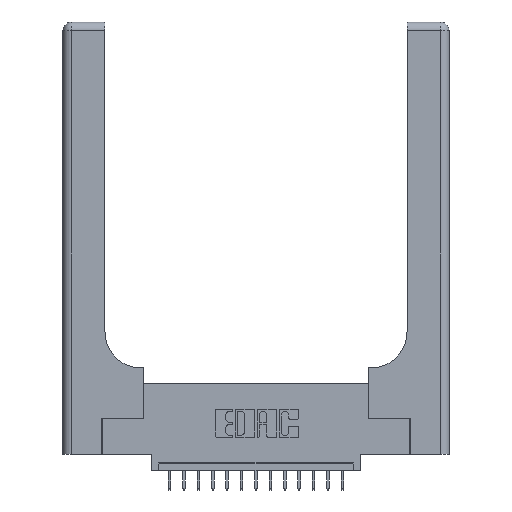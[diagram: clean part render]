
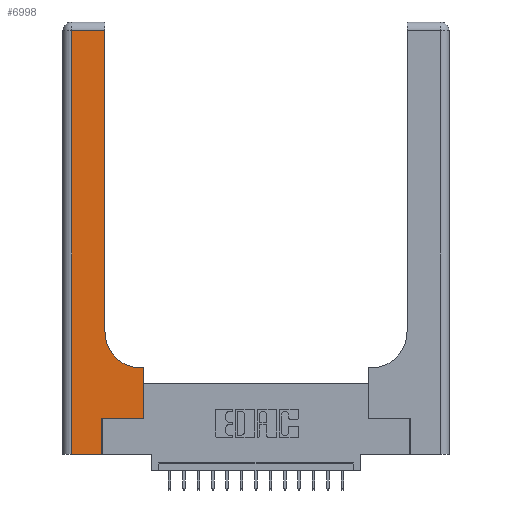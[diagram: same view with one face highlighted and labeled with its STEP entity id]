
A CAD part, top view. The second image highlights one B-rep face of the part: STEP entity #6998.
In plain terms, the highlighted planar face has unit normal (0, 0, 1).
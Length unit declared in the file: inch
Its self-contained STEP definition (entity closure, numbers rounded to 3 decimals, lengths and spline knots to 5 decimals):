
#561 = CARTESIAN_POINT ( 'NONE',  ( 0.269, 0.25, 0.37 ) ) ;
#608 = LINE ( 'NONE', #16810, #2091 ) ;
#616 = CARTESIAN_POINT ( 'NONE',  ( 0.2915, 2.94, 0.37 ) ) ;
#638 = LINE ( 'NONE', #5165, #14674 ) ;
#771 = ORIENTED_EDGE ( 'NONE', *, *, #9274, .T. ) ;
#991 = ORIENTED_EDGE ( 'NONE', *, *, #13420, .T. ) ;
#998 = ORIENTED_EDGE ( 'NONE', *, *, #8597, .T. ) ;
#1285 = DIRECTION ( 'NONE',  ( 1., 0., 0. ) ) ;
#1590 = CARTESIAN_POINT ( 'NONE',  ( 0., 2.94, 0.37 ) ) ;
#1772 = EDGE_CURVE ( 'NONE', #9181, #18291, #14982, .T. ) ;
#2091 = VECTOR ( 'NONE', #5419, 39.37008 ) ;
#2527 = FACE_OUTER_BOUND ( 'NONE', #10861, .T. ) ;
#2528 = CARTESIAN_POINT ( 'NONE',  ( 0.5585, 0.25, 0.37 ) ) ;
#2594 = EDGE_CURVE ( 'NONE', #7961, #16910, #15760, .T. ) ;
#2652 = CARTESIAN_POINT ( 'NONE',  ( 0., 0., 0.37 ) ) ;
#2973 = DIRECTION ( 'NONE',  ( 1., 0., 0. ) ) ;
#2987 = ORIENTED_EDGE ( 'NONE', *, *, #18652, .T. ) ;
#3195 = DIRECTION ( 'NONE',  ( 0., 1., 0. ) ) ;
#3884 = CIRCLE ( 'NONE', #10097, 0.25 ) ;
#4090 = LINE ( 'NONE', #9847, #17593 ) ;
#4193 = VERTEX_POINT ( 'NONE', #12497 ) ;
#4976 = CARTESIAN_POINT ( 'NONE',  ( 0.269, 0., 0.37 ) ) ;
#5077 = VECTOR ( 'NONE', #7003, 39.37008 ) ;
#5145 = CARTESIAN_POINT ( 'NONE',  ( 0.5585, 0.6, 0.37 ) ) ;
#5165 = CARTESIAN_POINT ( 'NONE',  ( 0.2915, 0.6, 0.37 ) ) ;
#5419 = DIRECTION ( 'NONE',  ( 0., 1., 0. ) ) ;
#5453 = VERTEX_POINT ( 'NONE', #616 ) ;
#6640 = AXIS2_PLACEMENT_3D ( 'NONE', #7092, #8457, #6906 ) ;
#6906 = DIRECTION ( 'NONE',  ( -1., 0., 0. ) ) ;
#6998 = ADVANCED_FACE ( 'NONE', ( #2527 ), #13167, .F. ) ;
#7003 = DIRECTION ( 'NONE',  ( 0., 1., 0. ) ) ;
#7092 = CARTESIAN_POINT ( 'NONE',  ( 0., 3., 0.37 ) ) ;
#7511 = DIRECTION ( 'NONE',  ( -1., 0., 0. ) ) ;
#7774 = VECTOR ( 'NONE', #7511, 39.37008 ) ;
#7961 = VERTEX_POINT ( 'NONE', #15566 ) ;
#8004 = DIRECTION ( 'NONE',  ( -1., 0., 0. ) ) ;
#8240 = CARTESIAN_POINT ( 'NONE',  ( 0.5415, 0.6, 0.37 ) ) ;
#8259 = ORIENTED_EDGE ( 'NONE', *, *, #2594, .T. ) ;
#8457 = DIRECTION ( 'NONE',  ( 0., 0., -1. ) ) ;
#8597 = EDGE_CURVE ( 'NONE', #17980, #13840, #3884, .T. ) ;
#8748 = VERTEX_POINT ( 'NONE', #13701 ) ;
#9069 = LINE ( 'NONE', #1590, #7774 ) ;
#9181 = VERTEX_POINT ( 'NONE', #4976 ) ;
#9274 = EDGE_CURVE ( 'NONE', #16910, #17980, #638, .T. ) ;
#9847 = CARTESIAN_POINT ( 'NONE',  ( 0.06, 3., 0.37 ) ) ;
#10097 = AXIS2_PLACEMENT_3D ( 'NONE', #13238, #10357, #2973 ) ;
#10357 = DIRECTION ( 'NONE',  ( 0., 0., -1. ) ) ;
#10702 = EDGE_CURVE ( 'NONE', #13840, #5453, #608, .T. ) ;
#10861 = EDGE_LOOP ( 'NONE', ( #15750, #2987, #13862, #991, #12794, #16191, #8259, #771, #998 ) ) ;
#11598 = LINE ( 'NONE', #14553, #17906 ) ;
#11784 = DIRECTION ( 'NONE',  ( 1., 0., 0. ) ) ;
#12497 = CARTESIAN_POINT ( 'NONE',  ( 0.06, 0., 0.37 ) ) ;
#12794 = ORIENTED_EDGE ( 'NONE', *, *, #1772, .T. ) ;
#13167 = PLANE ( 'NONE',  #6640 ) ;
#13190 = DIRECTION ( 'NONE',  ( 0., -1., 0. ) ) ;
#13238 = CARTESIAN_POINT ( 'NONE',  ( 0.5415, 0.85, 0.37 ) ) ;
#13420 = EDGE_CURVE ( 'NONE', #4193, #9181, #17399, .T. ) ;
#13701 = CARTESIAN_POINT ( 'NONE',  ( 0.06, 2.94, 0.37 ) ) ;
#13751 = VECTOR ( 'NONE', #3195, 39.37008 ) ;
#13840 = VERTEX_POINT ( 'NONE', #18362 ) ;
#13862 = ORIENTED_EDGE ( 'NONE', *, *, #18799, .T. ) ;
#14553 = CARTESIAN_POINT ( 'NONE',  ( 0.269, 0.25, 0.37 ) ) ;
#14674 = VECTOR ( 'NONE', #8004, 39.37008 ) ;
#14747 = VECTOR ( 'NONE', #1285, 39.37008 ) ;
#14982 = LINE ( 'NONE', #17874, #13751 ) ;
#15566 = CARTESIAN_POINT ( 'NONE',  ( 0.5585, 0.25, 0.37 ) ) ;
#15750 = ORIENTED_EDGE ( 'NONE', *, *, #10702, .T. ) ;
#15760 = LINE ( 'NONE', #2528, #5077 ) ;
#16191 = ORIENTED_EDGE ( 'NONE', *, *, #16291, .T. ) ;
#16291 = EDGE_CURVE ( 'NONE', #18291, #7961, #11598, .T. ) ;
#16810 = CARTESIAN_POINT ( 'NONE',  ( 0.2915, 3., 0.37 ) ) ;
#16910 = VERTEX_POINT ( 'NONE', #5145 ) ;
#17399 = LINE ( 'NONE', #2652, #14747 ) ;
#17593 = VECTOR ( 'NONE', #13190, 39.37008 ) ;
#17874 = CARTESIAN_POINT ( 'NONE',  ( 0.269, 0., 0.37 ) ) ;
#17906 = VECTOR ( 'NONE', #11784, 39.37008 ) ;
#17980 = VERTEX_POINT ( 'NONE', #8240 ) ;
#18291 = VERTEX_POINT ( 'NONE', #561 ) ;
#18362 = CARTESIAN_POINT ( 'NONE',  ( 0.2915, 0.85, 0.37 ) ) ;
#18652 = EDGE_CURVE ( 'NONE', #5453, #8748, #9069, .T. ) ;
#18799 = EDGE_CURVE ( 'NONE', #8748, #4193, #4090, .T. ) ;
